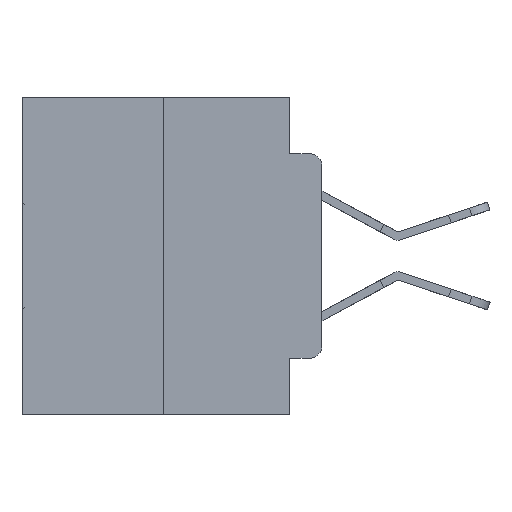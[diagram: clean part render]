
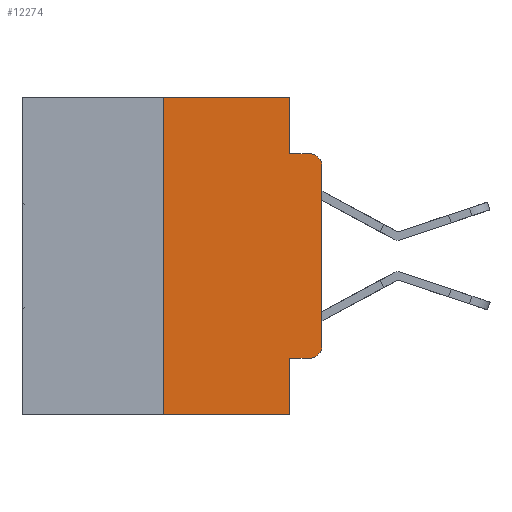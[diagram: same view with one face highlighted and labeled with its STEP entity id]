
A CAD part, left-side view. The second image highlights one B-rep face of the part: STEP entity #12274.
In plain terms, the highlighted planar face has unit normal (-1, 0, 0).
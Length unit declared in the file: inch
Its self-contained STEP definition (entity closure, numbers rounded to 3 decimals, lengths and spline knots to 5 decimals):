
#373 = ORIENTED_EDGE ( 'NONE', *, *, #30346, .F. ) ;
#755 = VERTEX_POINT ( 'NONE', #7376 ) ;
#1812 = EDGE_CURVE ( 'NONE', #10459, #19017, #20315, .T. ) ;
#1817 = EDGE_CURVE ( 'NONE', #17226, #26272, #8411, .T. ) ;
#3612 = DIRECTION ( 'NONE',  ( 0., -1., 0. ) ) ;
#3765 = CARTESIAN_POINT ( 'NONE',  ( 0., 0.051, 0. ) ) ;
#4044 = LINE ( 'NONE', #10779, #19404 ) ;
#4726 = CARTESIAN_POINT ( 'NONE',  ( 0., 0.473, 0. ) ) ;
#5185 = EDGE_CURVE ( 'NONE', #17226, #8176, #17026, .T. ) ;
#5496 = ORIENTED_EDGE ( 'NONE', *, *, #1812, .F. ) ;
#5670 = VERTEX_POINT ( 'NONE', #26197 ) ;
#6295 = CARTESIAN_POINT ( 'NONE',  ( 0., 0., -0.1085 ) ) ;
#6395 = EDGE_CURVE ( 'NONE', #10200, #20842, #8422, .T. ) ;
#6551 = DIRECTION ( 'NONE',  ( 0., 0., -1. ) ) ;
#6917 = DIRECTION ( 'NONE',  ( 0., 0., -1. ) ) ;
#7004 = ORIENTED_EDGE ( 'NONE', *, *, #5185, .F. ) ;
#7342 = CARTESIAN_POINT ( 'NONE',  ( 0., 0.02, -0.0885 ) ) ;
#7376 = CARTESIAN_POINT ( 'NONE',  ( 0., 0., -0.3915 ) ) ;
#7475 = CARTESIAN_POINT ( 'NONE',  ( 0., 0.25, 0. ) ) ;
#7992 = LINE ( 'NONE', #17679, #22188 ) ;
#8126 = CIRCLE ( 'NONE', #22817, 0.02 ) ;
#8176 = VERTEX_POINT ( 'NONE', #10653 ) ;
#8411 = LINE ( 'NONE', #27786, #10180 ) ;
#8422 = CIRCLE ( 'NONE', #30232, 0.02 ) ;
#9132 = ORIENTED_EDGE ( 'NONE', *, *, #10232, .T. ) ;
#9564 = DIRECTION ( 'NONE',  ( 0., -1., 0. ) ) ;
#10180 = VECTOR ( 'NONE', #3612, 39.37008 ) ;
#10200 = VERTEX_POINT ( 'NONE', #6295 ) ;
#10232 = EDGE_CURVE ( 'NONE', #755, #10200, #4044, .T. ) ;
#10459 = VERTEX_POINT ( 'NONE', #12494 ) ;
#10653 = CARTESIAN_POINT ( 'NONE',  ( 0., 0.25, 0. ) ) ;
#10779 = CARTESIAN_POINT ( 'NONE',  ( 0., 0., 0. ) ) ;
#11276 = EDGE_CURVE ( 'NONE', #19017, #20842, #24302, .T. ) ;
#12274 = ADVANCED_FACE ( 'NONE', ( #23294 ), #18535, .F. ) ;
#12494 = CARTESIAN_POINT ( 'NONE',  ( 0., 0.051, 0. ) ) ;
#13339 = CARTESIAN_POINT ( 'NONE',  ( 0., 0.02, -0.3915 ) ) ;
#13700 = VECTOR ( 'NONE', #29391, 39.37008 ) ;
#13789 = DIRECTION ( 'NONE',  ( 0., 0., 1. ) ) ;
#15213 = VERTEX_POINT ( 'NONE', #23307 ) ;
#15855 = DIRECTION ( 'NONE',  ( 1., 0., 0. ) ) ;
#16143 = CARTESIAN_POINT ( 'NONE',  ( 0., 0.051, -0.5 ) ) ;
#16219 = ORIENTED_EDGE ( 'NONE', *, *, #16690, .T. ) ;
#16628 = ORIENTED_EDGE ( 'NONE', *, *, #20161, .T. ) ;
#16665 = DIRECTION ( 'NONE',  ( 0., -1., 0. ) ) ;
#16690 = EDGE_CURVE ( 'NONE', #15213, #5670, #7992, .T. ) ;
#16857 = CARTESIAN_POINT ( 'NONE',  ( 0., 0.051, -0.0885 ) ) ;
#17026 = LINE ( 'NONE', #7475, #13700 ) ;
#17107 = ORIENTED_EDGE ( 'NONE', *, *, #6395, .T. ) ;
#17177 = EDGE_LOOP ( 'NONE', ( #9132, #17107, #30188, #5496, #373, #7004, #26088, #20994, #16219, #16628 ) ) ;
#17226 = VERTEX_POINT ( 'NONE', #28071 ) ;
#17679 = CARTESIAN_POINT ( 'NONE',  ( 0., 0.051, -0.4115 ) ) ;
#18336 = VECTOR ( 'NONE', #6917, 39.37008 ) ;
#18535 = PLANE ( 'NONE',  #21152 ) ;
#18892 = LINE ( 'NONE', #4726, #22947 ) ;
#19017 = VERTEX_POINT ( 'NONE', #28197 ) ;
#19404 = VECTOR ( 'NONE', #13789, 39.37008 ) ;
#20161 = EDGE_CURVE ( 'NONE', #5670, #755, #8126, .T. ) ;
#20315 = LINE ( 'NONE', #3765, #26365 ) ;
#20842 = VERTEX_POINT ( 'NONE', #7342 ) ;
#20994 = ORIENTED_EDGE ( 'NONE', *, *, #22105, .F. ) ;
#21152 = AXIS2_PLACEMENT_3D ( 'NONE', #28384, #15855, #28547 ) ;
#22105 = EDGE_CURVE ( 'NONE', #15213, #26272, #25816, .T. ) ;
#22188 = VECTOR ( 'NONE', #27359, 39.37008 ) ;
#22817 = AXIS2_PLACEMENT_3D ( 'NONE', #13339, #25695, #23012 ) ;
#22947 = VECTOR ( 'NONE', #16665, 39.37008 ) ;
#23012 = DIRECTION ( 'NONE',  ( 0., 0., -1. ) ) ;
#23294 = FACE_OUTER_BOUND ( 'NONE', #17177, .T. ) ;
#23307 = CARTESIAN_POINT ( 'NONE',  ( 0., 0.051, -0.4115 ) ) ;
#23764 = CARTESIAN_POINT ( 'NONE',  ( 0., 0.051, 0. ) ) ;
#24282 = VECTOR ( 'NONE', #9564, 39.37008 ) ;
#24302 = LINE ( 'NONE', #16857, #24282 ) ;
#25392 = DIRECTION ( 'NONE',  ( 0., 0., -1. ) ) ;
#25695 = DIRECTION ( 'NONE',  ( -1., 0., 0. ) ) ;
#25816 = LINE ( 'NONE', #23764, #18336 ) ;
#26088 = ORIENTED_EDGE ( 'NONE', *, *, #1817, .T. ) ;
#26089 = DIRECTION ( 'NONE',  ( -1., 0., 0. ) ) ;
#26197 = CARTESIAN_POINT ( 'NONE',  ( 0., 0.02, -0.4115 ) ) ;
#26272 = VERTEX_POINT ( 'NONE', #16143 ) ;
#26365 = VECTOR ( 'NONE', #25392, 39.37008 ) ;
#27359 = DIRECTION ( 'NONE',  ( 0., -1., 0. ) ) ;
#27786 = CARTESIAN_POINT ( 'NONE',  ( 0., 0.473, -0.5 ) ) ;
#28071 = CARTESIAN_POINT ( 'NONE',  ( 0., 0.25, -0.5 ) ) ;
#28197 = CARTESIAN_POINT ( 'NONE',  ( 0., 0.051, -0.0885 ) ) ;
#28384 = CARTESIAN_POINT ( 'NONE',  ( 0., 0.473, 0. ) ) ;
#28547 = DIRECTION ( 'NONE',  ( 0., 0., -1. ) ) ;
#29391 = DIRECTION ( 'NONE',  ( 0., 0., 1. ) ) ;
#30188 = ORIENTED_EDGE ( 'NONE', *, *, #11276, .F. ) ;
#30232 = AXIS2_PLACEMENT_3D ( 'NONE', #31172, #26089, #6551 ) ;
#30346 = EDGE_CURVE ( 'NONE', #8176, #10459, #18892, .T. ) ;
#31172 = CARTESIAN_POINT ( 'NONE',  ( 0., 0.02, -0.1085 ) ) ;
